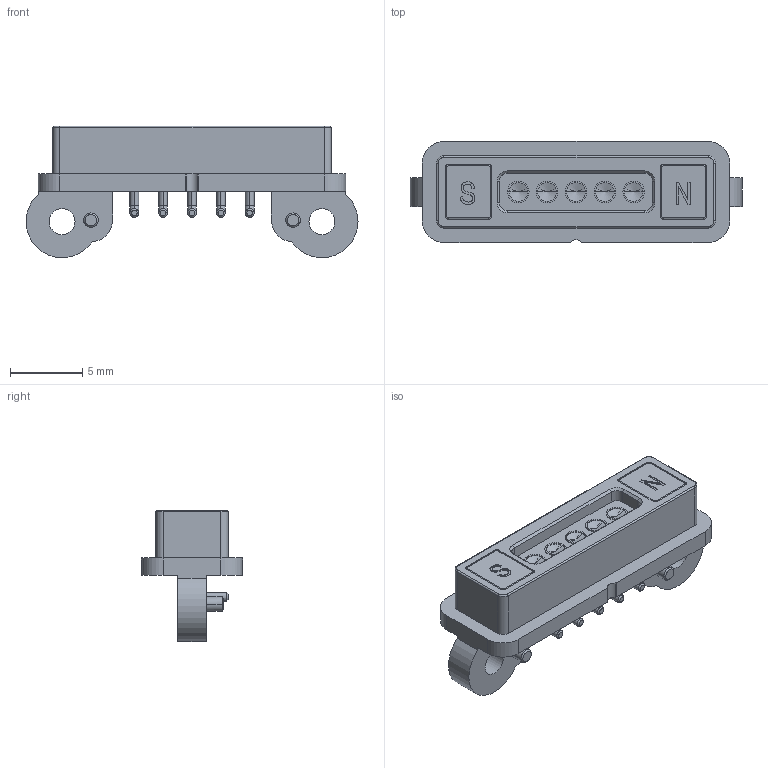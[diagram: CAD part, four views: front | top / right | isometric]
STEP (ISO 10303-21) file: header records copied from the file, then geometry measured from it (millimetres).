
FILE_DESCRIPTION (( 'STEP AP214' ), '1' );
FILE_NAME ('686J0521350124E.STEP', '2023-04-13T18:51:59', ( '' ), ( '' ), 'SwSTEP 2.0', 'SolidWorks 2020', '' );
FILE_SCHEMA (( 'AUTOMOTIVE_DESIGN' ));
Length unit declared in the file: millimetre
Products named in the file (1): 686J0521350124E
Bounding box: 23 x 7 x 9.1 mm (x, y, z)
Volume: 515.2 mm3; surface area: 840.1 mm2
Topology: 6 solids, 8 shells, 303 faces, 698 edges, 428 vertices
Faces by surface type: cylinder 124, plane 103, cone 32, bspline 26, torus 18
Entity records: 12709 total; most frequent: CARTESIAN_POINT 2482, DIRECTION 1499, ORIENTED_EDGE 1376, EDGE_CURVE 688, AXIS2_PLACEMENT_3D 573, VERTEX_POINT 428, LINE 353, VECTOR 353
